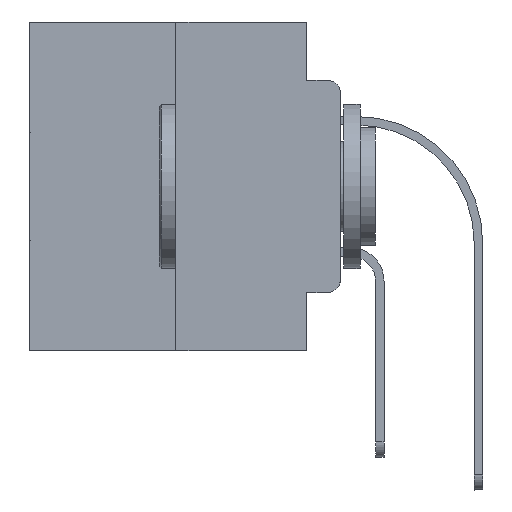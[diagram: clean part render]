
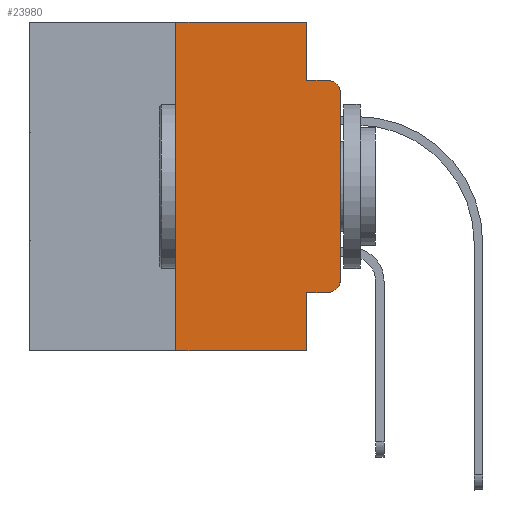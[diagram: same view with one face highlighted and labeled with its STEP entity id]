
A CAD part, left-side view. The second image highlights one B-rep face of the part: STEP entity #23980.
In plain terms, the highlighted planar face has unit normal (-1, 0, 0).
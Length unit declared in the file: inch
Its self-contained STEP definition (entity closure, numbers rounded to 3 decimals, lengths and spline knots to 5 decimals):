
#356 = VECTOR ( 'NONE', #8413, 39.37008 ) ;
#1000 = CARTESIAN_POINT ( 'NONE',  ( 0., 0., 0. ) ) ;
#1021 = CARTESIAN_POINT ( 'NONE',  ( 0., 0.02, -0.3915 ) ) ;
#2046 = CARTESIAN_POINT ( 'NONE',  ( 0., 0.25, 0. ) ) ;
#2059 = VECTOR ( 'NONE', #24969, 39.37008 ) ;
#2505 = DIRECTION ( 'NONE',  ( 1., 0., 0. ) ) ;
#2713 = VECTOR ( 'NONE', #27249, 39.37008 ) ;
#3372 = CARTESIAN_POINT ( 'NONE',  ( 0., 0.051, -0.4115 ) ) ;
#3593 = CARTESIAN_POINT ( 'NONE',  ( 0., 0.051, -0.0885 ) ) ;
#3635 = DIRECTION ( 'NONE',  ( 0., 0., -1. ) ) ;
#4446 = CARTESIAN_POINT ( 'NONE',  ( 0., 0., -0.1085 ) ) ;
#4525 = PLANE ( 'NONE',  #27238 ) ;
#4538 = LINE ( 'NONE', #29882, #18692 ) ;
#5326 = ORIENTED_EDGE ( 'NONE', *, *, #11716, .F. ) ;
#5641 = LINE ( 'NONE', #1000, #2713 ) ;
#6239 = VECTOR ( 'NONE', #7899, 39.37008 ) ;
#6352 = VERTEX_POINT ( 'NONE', #24386 ) ;
#7574 = CARTESIAN_POINT ( 'NONE',  ( 0., 0.051, 0. ) ) ;
#7899 = DIRECTION ( 'NONE',  ( 0., -1., 0. ) ) ;
#8101 = ORIENTED_EDGE ( 'NONE', *, *, #23893, .F. ) ;
#8413 = DIRECTION ( 'NONE',  ( 0., -1., 0. ) ) ;
#8638 = VERTEX_POINT ( 'NONE', #3372 ) ;
#9024 = LINE ( 'NONE', #3593, #12846 ) ;
#10217 = LINE ( 'NONE', #19693, #6239 ) ;
#10228 = ORIENTED_EDGE ( 'NONE', *, *, #18014, .F. ) ;
#11292 = VERTEX_POINT ( 'NONE', #29370 ) ;
#11635 = VERTEX_POINT ( 'NONE', #15036 ) ;
#11716 = EDGE_CURVE ( 'NONE', #23997, #22713, #10217, .T. ) ;
#11745 = ORIENTED_EDGE ( 'NONE', *, *, #23437, .T. ) ;
#12587 = EDGE_CURVE ( 'NONE', #27236, #6352, #25623, .T. ) ;
#12846 = VECTOR ( 'NONE', #29870, 39.37008 ) ;
#13849 = CARTESIAN_POINT ( 'NONE',  ( 0., 0., -0.3915 ) ) ;
#13883 = CIRCLE ( 'NONE', #26289, 0.02 ) ;
#13999 = CARTESIAN_POINT ( 'NONE',  ( 0., 0.473, 0. ) ) ;
#14045 = CARTESIAN_POINT ( 'NONE',  ( 0., 0.25, -0.5 ) ) ;
#14303 = VECTOR ( 'NONE', #25242, 39.37008 ) ;
#15036 = CARTESIAN_POINT ( 'NONE',  ( 0., 0.02, -0.4115 ) ) ;
#15246 = CARTESIAN_POINT ( 'NONE',  ( 0., 0.051, -0.4115 ) ) ;
#15655 = VERTEX_POINT ( 'NONE', #14045 ) ;
#15679 = DIRECTION ( 'NONE',  ( 0., 0., -1. ) ) ;
#15698 = ORIENTED_EDGE ( 'NONE', *, *, #16059, .F. ) ;
#16059 = EDGE_CURVE ( 'NONE', #15655, #23997, #27982, .T. ) ;
#16472 = FACE_OUTER_BOUND ( 'NONE', #22586, .T. ) ;
#16854 = VECTOR ( 'NONE', #26293, 39.37008 ) ;
#17977 = CARTESIAN_POINT ( 'NONE',  ( 0., 0.051, -0.5 ) ) ;
#17992 = LINE ( 'NONE', #27313, #2059 ) ;
#18014 = EDGE_CURVE ( 'NONE', #8638, #21740, #17992, .T. ) ;
#18022 = CARTESIAN_POINT ( 'NONE',  ( 0., 0.02, -0.1085 ) ) ;
#18692 = VECTOR ( 'NONE', #30191, 39.37008 ) ;
#19693 = CARTESIAN_POINT ( 'NONE',  ( 0., 0.473, 0. ) ) ;
#20342 = DIRECTION ( 'NONE',  ( -1., 0., 0. ) ) ;
#20426 = EDGE_CURVE ( 'NONE', #22713, #11292, #4538, .T. ) ;
#21740 = VERTEX_POINT ( 'NONE', #17977 ) ;
#22586 = EDGE_LOOP ( 'NONE', ( #26269, #28090, #8101, #25639, #5326, #15698, #11745, #10228, #26274, #25563 ) ) ;
#22588 = DIRECTION ( 'NONE',  ( -1., 0., 0. ) ) ;
#22713 = VERTEX_POINT ( 'NONE', #7574 ) ;
#23437 = EDGE_CURVE ( 'NONE', #15655, #21740, #29755, .T. ) ;
#23893 = EDGE_CURVE ( 'NONE', #11292, #6352, #9024, .T. ) ;
#23980 = ADVANCED_FACE ( 'NONE', ( #16472 ), #4525, .F. ) ;
#23997 = VERTEX_POINT ( 'NONE', #2046 ) ;
#24386 = CARTESIAN_POINT ( 'NONE',  ( 0., 0.02, -0.0885 ) ) ;
#24616 = EDGE_CURVE ( 'NONE', #11635, #29314, #13883, .T. ) ;
#24969 = DIRECTION ( 'NONE',  ( 0., 0., -1. ) ) ;
#25242 = DIRECTION ( 'NONE',  ( 0., -1., 0. ) ) ;
#25563 = ORIENTED_EDGE ( 'NONE', *, *, #24616, .T. ) ;
#25623 = CIRCLE ( 'NONE', #27622, 0.02 ) ;
#25639 = ORIENTED_EDGE ( 'NONE', *, *, #20426, .F. ) ;
#25952 = DIRECTION ( 'NONE',  ( 0., 0., -1. ) ) ;
#26183 = EDGE_CURVE ( 'NONE', #29314, #27236, #5641, .T. ) ;
#26269 = ORIENTED_EDGE ( 'NONE', *, *, #26183, .T. ) ;
#26274 = ORIENTED_EDGE ( 'NONE', *, *, #27964, .T. ) ;
#26289 = AXIS2_PLACEMENT_3D ( 'NONE', #1021, #22588, #3635 ) ;
#26293 = DIRECTION ( 'NONE',  ( 0., 0., 1. ) ) ;
#27236 = VERTEX_POINT ( 'NONE', #4446 ) ;
#27238 = AXIS2_PLACEMENT_3D ( 'NONE', #13999, #2505, #25952 ) ;
#27249 = DIRECTION ( 'NONE',  ( 0., 0., 1. ) ) ;
#27313 = CARTESIAN_POINT ( 'NONE',  ( 0., 0.051, 0. ) ) ;
#27622 = AXIS2_PLACEMENT_3D ( 'NONE', #18022, #20342, #15679 ) ;
#27964 = EDGE_CURVE ( 'NONE', #8638, #11635, #29710, .T. ) ;
#27982 = LINE ( 'NONE', #28148, #16854 ) ;
#28090 = ORIENTED_EDGE ( 'NONE', *, *, #12587, .T. ) ;
#28148 = CARTESIAN_POINT ( 'NONE',  ( 0., 0.25, 0. ) ) ;
#29314 = VERTEX_POINT ( 'NONE', #13849 ) ;
#29370 = CARTESIAN_POINT ( 'NONE',  ( 0., 0.051, -0.0885 ) ) ;
#29710 = LINE ( 'NONE', #15246, #356 ) ;
#29755 = LINE ( 'NONE', #30356, #14303 ) ;
#29870 = DIRECTION ( 'NONE',  ( 0., -1., 0. ) ) ;
#29882 = CARTESIAN_POINT ( 'NONE',  ( 0., 0.051, 0. ) ) ;
#30191 = DIRECTION ( 'NONE',  ( 0., 0., -1. ) ) ;
#30356 = CARTESIAN_POINT ( 'NONE',  ( 0., 0.473, -0.5 ) ) ;
